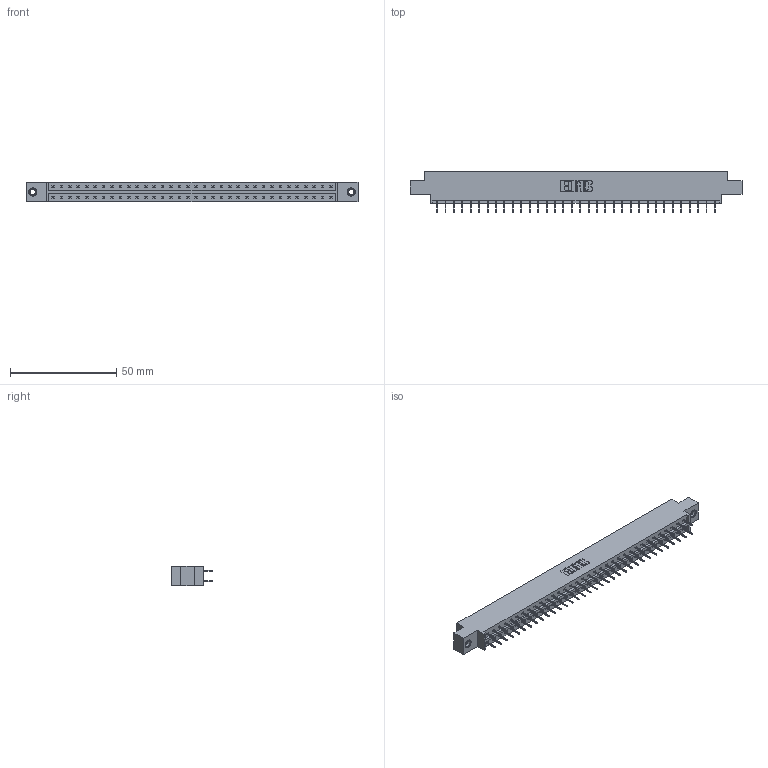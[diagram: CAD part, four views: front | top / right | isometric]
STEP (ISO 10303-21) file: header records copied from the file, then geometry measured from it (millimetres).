
FILE_DESCRIPTION (( 'STEP AP203' ), '1' );
FILE_NAME ('333-068-524-807.STEP', '2018-08-04T12:53:09', ( '' ), ( '' ), 'SwSTEP 2.0', 'SolidWorks 2016', '' );
FILE_SCHEMA (( 'CONFIG_CONTROL_DESIGN' ));
Length unit declared in the file: inch
Products named in the file (4): 333-068-524-807; 333 Part_Offset - .156 Dia - TI; 345-292-001_345-293-124; 345-250-001_345-250-005-103
Assembly tree (71 placements, depth 2):
  333-068-524-807
    333 Part_Offset - .156 Dia - TI
    345-292-001_345-293-124  x68
    345-250-001_345-250-005-103  x2
Bounding box: 156.26 x 19.69 x 9.4 mm (x, y, z)
Volume: 15534.3 mm3; surface area: 18225.6 mm2
Topology: 71 solids, 71 shells, 3986 faces, 11271 edges, 7234 vertices
Faces by surface type: plane 2962, cylinder 1008, cone 12, torus 4
Entity records: 24300 total; most frequent: CARTESIAN_POINT 4021, ORIENTED_EDGE 3950, DIRECTION 3481, EDGE_CURVE 1975, LINE 1831, VECTOR 1831, VERTEX_POINT 1308, AXIS2_PLACEMENT_3D 825
